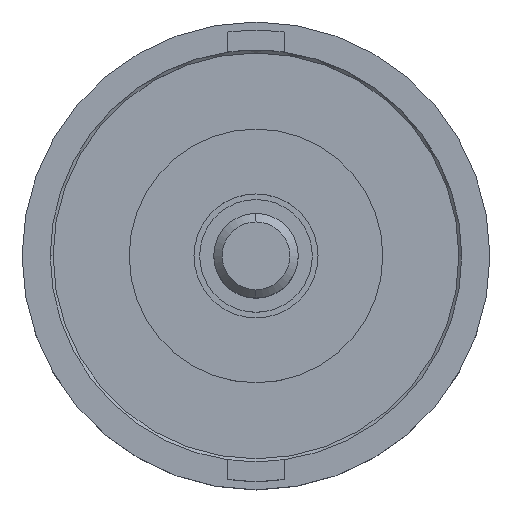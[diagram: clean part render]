
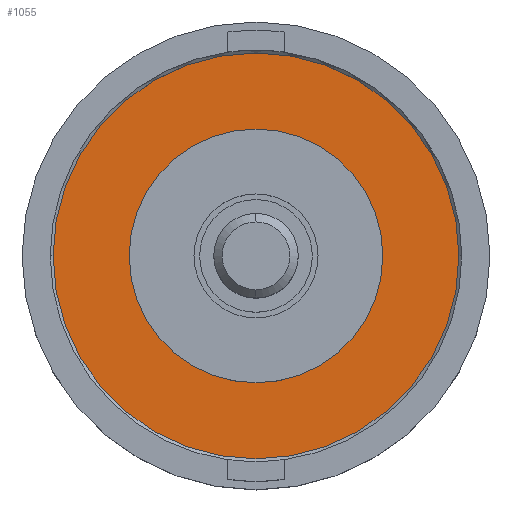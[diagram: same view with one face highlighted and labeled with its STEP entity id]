
A CAD part, top view. The second image highlights one B-rep face of the part: STEP entity #1055.
In plain terms, the highlighted planar face has unit normal (0, 0, 1).
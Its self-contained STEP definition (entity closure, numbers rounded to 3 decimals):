
#96 = DIRECTION ( 'NONE',  ( -1., 0., 0. ) ) ;
#123 = CARTESIAN_POINT ( 'NONE',  ( -3.6, 0., 9.65 ) ) ;
#149 = EDGE_LOOP ( 'NONE', ( #674, #563 ) ) ;
#154 = EDGE_CURVE ( 'NONE', #308, #225, #1295, .T. ) ;
#206 = AXIS2_PLACEMENT_3D ( 'NONE', #1360, #1480, #1130 ) ;
#207 = ORIENTED_EDGE ( 'NONE', *, *, #1358, .T. ) ;
#225 = VERTEX_POINT ( 'NONE', #444 ) ;
#238 = PLANE ( 'NONE',  #813 ) ;
#247 = DIRECTION ( 'NONE',  ( 0., 0., -1. ) ) ;
#255 = CARTESIAN_POINT ( 'NONE',  ( -2.25, 0., 9.65 ) ) ;
#306 = DIRECTION ( 'NONE',  ( 0., 0., 1. ) ) ;
#308 = VERTEX_POINT ( 'NONE', #255 ) ;
#314 = CARTESIAN_POINT ( 'NONE',  ( 0., 0., 9.65 ) ) ;
#437 = DIRECTION ( 'NONE',  ( 0., 0., -1. ) ) ;
#441 = DIRECTION ( 'NONE',  ( 0., 0., 1. ) ) ;
#444 = CARTESIAN_POINT ( 'NONE',  ( 2.25, 0., 9.65 ) ) ;
#552 = AXIS2_PLACEMENT_3D ( 'NONE', #705, #247, #1182 ) ;
#563 = ORIENTED_EDGE ( 'NONE', *, *, #721, .T. ) ;
#564 = DIRECTION ( 'NONE',  ( 1., 0., 0. ) ) ;
#586 = FACE_OUTER_BOUND ( 'NONE', #1379, .T. ) ;
#674 = ORIENTED_EDGE ( 'NONE', *, *, #154, .T. ) ;
#678 = AXIS2_PLACEMENT_3D ( 'NONE', #1144, #437, #96 ) ;
#705 = CARTESIAN_POINT ( 'NONE',  ( 0., 0., 9.65 ) ) ;
#721 = EDGE_CURVE ( 'NONE', #225, #308, #1488, .T. ) ;
#740 = AXIS2_PLACEMENT_3D ( 'NONE', #314, #306, #1014 ) ;
#779 = ORIENTED_EDGE ( 'NONE', *, *, #1298, .T. ) ;
#813 = AXIS2_PLACEMENT_3D ( 'NONE', #1040, #441, #564 ) ;
#1014 = DIRECTION ( 'NONE',  ( -1., 0., 0. ) ) ;
#1040 = CARTESIAN_POINT ( 'NONE',  ( 0., 0., 9.65 ) ) ;
#1055 = ADVANCED_FACE ( 'NONE', ( #1297, #586 ), #238, .T. ) ;
#1065 = VERTEX_POINT ( 'NONE', #123 ) ;
#1130 = DIRECTION ( 'NONE',  ( 1., 0., 0. ) ) ;
#1144 = CARTESIAN_POINT ( 'NONE',  ( 0., 0., 9.65 ) ) ;
#1182 = DIRECTION ( 'NONE',  ( 1., 0., 0. ) ) ;
#1225 = VERTEX_POINT ( 'NONE', #1441 ) ;
#1232 = CIRCLE ( 'NONE', #206, 3.6 ) ;
#1295 = CIRCLE ( 'NONE', #678, 2.25 ) ;
#1297 = FACE_BOUND ( 'NONE', #149, .T. ) ;
#1298 = EDGE_CURVE ( 'NONE', #1065, #1225, #1381, .T. ) ;
#1358 = EDGE_CURVE ( 'NONE', #1225, #1065, #1232, .T. ) ;
#1360 = CARTESIAN_POINT ( 'NONE',  ( 0., 0., 9.65 ) ) ;
#1379 = EDGE_LOOP ( 'NONE', ( #779, #207 ) ) ;
#1381 = CIRCLE ( 'NONE', #740, 3.6 ) ;
#1441 = CARTESIAN_POINT ( 'NONE',  ( 3.6, 0., 9.65 ) ) ;
#1480 = DIRECTION ( 'NONE',  ( 0., 0., 1. ) ) ;
#1488 = CIRCLE ( 'NONE', #552, 2.25 ) ;
